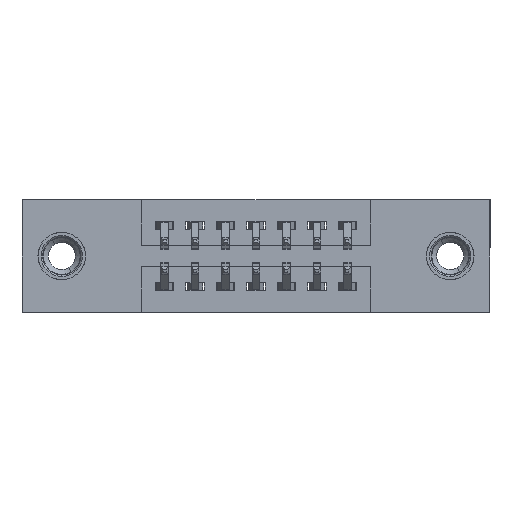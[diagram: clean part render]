
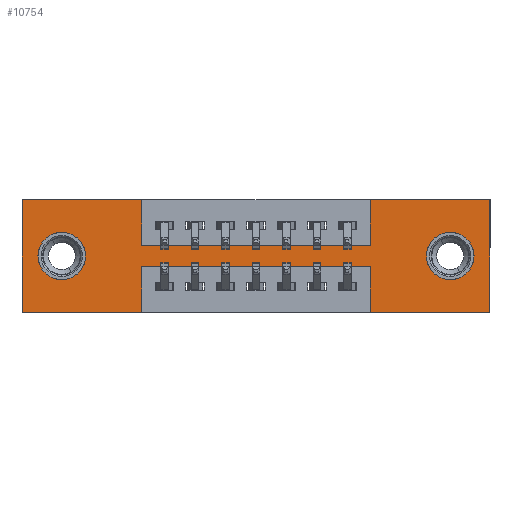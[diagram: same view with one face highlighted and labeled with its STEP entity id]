
A CAD part, front view. The second image highlights one B-rep face of the part: STEP entity #10754.
In plain terms, the highlighted planar face has unit normal (0, -1, 0).
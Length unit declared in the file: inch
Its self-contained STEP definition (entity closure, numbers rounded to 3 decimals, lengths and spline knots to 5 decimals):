
#37 = DIRECTION ( 'NONE',  ( 0., 1., 0. ) ) ;
#126 = DIRECTION ( 'NONE',  ( 0., 0., 1. ) ) ;
#140 = CARTESIAN_POINT ( 'NONE',  ( 0., 0., -0.37 ) ) ;
#160 = CARTESIAN_POINT ( 'NONE',  ( 1.1425, 0., -0.37 ) ) ;
#233 = VERTEX_POINT ( 'NONE', #1123 ) ;
#280 = DIRECTION ( 'NONE',  ( 0., 0., -1. ) ) ;
#320 = LINE ( 'NONE', #11896, #3684 ) ;
#445 = ORIENTED_EDGE ( 'NONE', *, *, #13156, .F. ) ;
#473 = ORIENTED_EDGE ( 'NONE', *, *, #13990, .F. ) ;
#594 = VECTOR ( 'NONE', #12571, 39.37008 ) ;
#724 = VERTEX_POINT ( 'NONE', #12053 ) ;
#751 = EDGE_LOOP ( 'NONE', ( #2129, #831 ) ) ;
#767 = ORIENTED_EDGE ( 'NONE', *, *, #3498, .T. ) ;
#792 = CARTESIAN_POINT ( 'NONE',  ( 0.3925, 0., -0.37 ) ) ;
#831 = ORIENTED_EDGE ( 'NONE', *, *, #5526, .T. ) ;
#1032 = ORIENTED_EDGE ( 'NONE', *, *, #11432, .F. ) ;
#1123 = CARTESIAN_POINT ( 'NONE',  ( 1.1425, 0., -0.15 ) ) ;
#1254 = CARTESIAN_POINT ( 'NONE',  ( 0., 0., 0. ) ) ;
#1284 = ORIENTED_EDGE ( 'NONE', *, *, #15122, .F. ) ;
#1580 = LINE ( 'NONE', #1654, #10946 ) ;
#1654 = CARTESIAN_POINT ( 'NONE',  ( 0.3925, 0., -0.22 ) ) ;
#1735 = LINE ( 'NONE', #140, #10733 ) ;
#1792 = VERTEX_POINT ( 'NONE', #6882 ) ;
#1902 = CARTESIAN_POINT ( 'NONE',  ( 0.3925, 0., 0. ) ) ;
#2129 = ORIENTED_EDGE ( 'NONE', *, *, #14119, .T. ) ;
#2216 = AXIS2_PLACEMENT_3D ( 'NONE', #4297, #10157, #3163 ) ;
#2231 = EDGE_CURVE ( 'NONE', #6655, #9765, #9321, .T. ) ;
#2238 = ORIENTED_EDGE ( 'NONE', *, *, #10975, .F. ) ;
#2498 = VECTOR ( 'NONE', #12984, 39.37008 ) ;
#2503 = VERTEX_POINT ( 'NONE', #13087 ) ;
#2559 = VERTEX_POINT ( 'NONE', #5867 ) ;
#2939 = LINE ( 'NONE', #14833, #11498 ) ;
#3027 = CARTESIAN_POINT ( 'NONE',  ( 0., 0., 0. ) ) ;
#3074 = EDGE_CURVE ( 'NONE', #1792, #12437, #1735, .T. ) ;
#3163 = DIRECTION ( 'NONE',  ( 0., 0., -1. ) ) ;
#3257 = LINE ( 'NONE', #14466, #6117 ) ;
#3259 = ORIENTED_EDGE ( 'NONE', *, *, #11015, .T. ) ;
#3344 = CARTESIAN_POINT ( 'NONE',  ( 0.13, 0., -0.263 ) ) ;
#3498 = EDGE_CURVE ( 'NONE', #9785, #724, #6095, .T. ) ;
#3549 = VECTOR ( 'NONE', #12951, 39.37008 ) ;
#3595 = ORIENTED_EDGE ( 'NONE', *, *, #13204, .F. ) ;
#3684 = VECTOR ( 'NONE', #5049, 39.37008 ) ;
#3766 = FACE_BOUND ( 'NONE', #751, .T. ) ;
#3791 = EDGE_CURVE ( 'NONE', #233, #10198, #3257, .T. ) ;
#4177 = CARTESIAN_POINT ( 'NONE',  ( 0.3925, 0., -0.15 ) ) ;
#4223 = DIRECTION ( 'NONE',  ( 0., 1., 0. ) ) ;
#4297 = CARTESIAN_POINT ( 'NONE',  ( 0., 0., -0.37 ) ) ;
#4320 = LINE ( 'NONE', #10291, #594 ) ;
#4828 = CARTESIAN_POINT ( 'NONE',  ( 1.1425, 0., -0.37 ) ) ;
#4930 = CARTESIAN_POINT ( 'NONE',  ( 0.13, 0., -0.185 ) ) ;
#4999 = ORIENTED_EDGE ( 'NONE', *, *, #3074, .F. ) ;
#5049 = DIRECTION ( 'NONE',  ( 0., 0., -1. ) ) ;
#5526 = EDGE_CURVE ( 'NONE', #5575, #7166, #11406, .T. ) ;
#5575 = VERTEX_POINT ( 'NONE', #7829 ) ;
#5647 = CARTESIAN_POINT ( 'NONE',  ( 0., 0., 0. ) ) ;
#5775 = CARTESIAN_POINT ( 'NONE',  ( 1.405, 0., -0.107 ) ) ;
#5867 = CARTESIAN_POINT ( 'NONE',  ( 1.535, 0., -0.37 ) ) ;
#6095 = CIRCLE ( 'NONE', #7546, 0.078 ) ;
#6117 = VECTOR ( 'NONE', #11138, 39.37008 ) ;
#6133 = DIRECTION ( 'NONE',  ( 0., 0., 1. ) ) ;
#6165 = VECTOR ( 'NONE', #9163, 39.37008 ) ;
#6533 = AXIS2_PLACEMENT_3D ( 'NONE', #14329, #7609, #280 ) ;
#6598 = LINE ( 'NONE', #792, #6165 ) ;
#6655 = VERTEX_POINT ( 'NONE', #4828 ) ;
#6708 = DIRECTION ( 'NONE',  ( 0., 0., -1. ) ) ;
#6790 = DIRECTION ( 'NONE',  ( -1., 0., 0. ) ) ;
#6882 = CARTESIAN_POINT ( 'NONE',  ( 0.3925, 0., -0.37 ) ) ;
#6951 = FACE_BOUND ( 'NONE', #11515, .T. ) ;
#7166 = VERTEX_POINT ( 'NONE', #5775 ) ;
#7375 = AXIS2_PLACEMENT_3D ( 'NONE', #11141, #4223, #12263 ) ;
#7396 = CARTESIAN_POINT ( 'NONE',  ( 0.13, 0., -0.185 ) ) ;
#7546 = AXIS2_PLACEMENT_3D ( 'NONE', #4930, #12903, #6133 ) ;
#7609 = DIRECTION ( 'NONE',  ( 0., 1., 0. ) ) ;
#7813 = DIRECTION ( 'NONE',  ( 1., 0., 0. ) ) ;
#7829 = CARTESIAN_POINT ( 'NONE',  ( 1.405, 0., -0.263 ) ) ;
#8384 = CARTESIAN_POINT ( 'NONE',  ( 1.535, 0., 0. ) ) ;
#8513 = VERTEX_POINT ( 'NONE', #4177 ) ;
#8518 = DIRECTION ( 'NONE',  ( 0., 0., 1. ) ) ;
#8630 = VECTOR ( 'NONE', #126, 39.37008 ) ;
#8665 = VECTOR ( 'NONE', #6708, 39.37008 ) ;
#8810 = VERTEX_POINT ( 'NONE', #8384 ) ;
#8982 = CARTESIAN_POINT ( 'NONE',  ( 1.1425, 0., 0. ) ) ;
#9163 = DIRECTION ( 'NONE',  ( 0., 0., -1. ) ) ;
#9321 = LINE ( 'NONE', #160, #8630 ) ;
#9758 = LINE ( 'NONE', #1254, #3549 ) ;
#9765 = VERTEX_POINT ( 'NONE', #13679 ) ;
#9785 = VERTEX_POINT ( 'NONE', #3344 ) ;
#9891 = ORIENTED_EDGE ( 'NONE', *, *, #13495, .F. ) ;
#9950 = FACE_OUTER_BOUND ( 'NONE', #11620, .T. ) ;
#10157 = DIRECTION ( 'NONE',  ( 0., -1., 0. ) ) ;
#10166 = EDGE_CURVE ( 'NONE', #10230, #10204, #14355, .T. ) ;
#10198 = VERTEX_POINT ( 'NONE', #8982 ) ;
#10204 = VERTEX_POINT ( 'NONE', #1902 ) ;
#10230 = VERTEX_POINT ( 'NONE', #5647 ) ;
#10291 = CARTESIAN_POINT ( 'NONE',  ( 0., 0., -0.37 ) ) ;
#10733 = VECTOR ( 'NONE', #6790, 39.37008 ) ;
#10754 = ADVANCED_FACE ( 'NONE', ( #3766, #6951, #9950 ), #14640, .T. ) ;
#10946 = VECTOR ( 'NONE', #13266, 39.37008 ) ;
#10975 = EDGE_CURVE ( 'NONE', #10198, #8810, #9758, .T. ) ;
#11015 = EDGE_CURVE ( 'NONE', #724, #9785, #12742, .T. ) ;
#11109 = CIRCLE ( 'NONE', #6533, 0.078 ) ;
#11138 = DIRECTION ( 'NONE',  ( 0., 0., 1. ) ) ;
#11141 = CARTESIAN_POINT ( 'NONE',  ( 1.405, 0., -0.185 ) ) ;
#11406 = CIRCLE ( 'NONE', #7375, 0.078 ) ;
#11432 = EDGE_CURVE ( 'NONE', #2559, #6655, #4320, .T. ) ;
#11498 = VECTOR ( 'NONE', #12566, 39.37008 ) ;
#11515 = EDGE_LOOP ( 'NONE', ( #3259, #767 ) ) ;
#11620 = EDGE_LOOP ( 'NONE', ( #3595, #9891, #11717, #1032, #473, #2238, #12476, #12797, #445, #13026, #1284, #4999 ) ) ;
#11717 = ORIENTED_EDGE ( 'NONE', *, *, #2231, .F. ) ;
#11896 = CARTESIAN_POINT ( 'NONE',  ( 1.535, 0., 0. ) ) ;
#12053 = CARTESIAN_POINT ( 'NONE',  ( 0.13, 0., -0.107 ) ) ;
#12263 = DIRECTION ( 'NONE',  ( 0., 0., -1. ) ) ;
#12437 = VERTEX_POINT ( 'NONE', #14450 ) ;
#12471 = CARTESIAN_POINT ( 'NONE',  ( 0.3925, 0., 0. ) ) ;
#12476 = ORIENTED_EDGE ( 'NONE', *, *, #3791, .F. ) ;
#12566 = DIRECTION ( 'NONE',  ( 1., 0., 0. ) ) ;
#12571 = DIRECTION ( 'NONE',  ( -1., 0., 0. ) ) ;
#12742 = CIRCLE ( 'NONE', #13116, 0.078 ) ;
#12797 = ORIENTED_EDGE ( 'NONE', *, *, #13251, .F. ) ;
#12903 = DIRECTION ( 'NONE',  ( 0., 1., 0. ) ) ;
#12951 = DIRECTION ( 'NONE',  ( 1., 0., 0. ) ) ;
#12984 = DIRECTION ( 'NONE',  ( 0., 0., 1. ) ) ;
#13026 = ORIENTED_EDGE ( 'NONE', *, *, #10166, .F. ) ;
#13087 = CARTESIAN_POINT ( 'NONE',  ( 0.3925, 0., -0.22 ) ) ;
#13116 = AXIS2_PLACEMENT_3D ( 'NONE', #7396, #37, #8518 ) ;
#13156 = EDGE_CURVE ( 'NONE', #10204, #8513, #14661, .T. ) ;
#13204 = EDGE_CURVE ( 'NONE', #2503, #1792, #6598, .T. ) ;
#13251 = EDGE_CURVE ( 'NONE', #8513, #233, #2939, .T. ) ;
#13266 = DIRECTION ( 'NONE',  ( -1., 0., 0. ) ) ;
#13495 = EDGE_CURVE ( 'NONE', #9765, #2503, #1580, .T. ) ;
#13679 = CARTESIAN_POINT ( 'NONE',  ( 1.1425, 0., -0.22 ) ) ;
#13713 = LINE ( 'NONE', #14066, #2498 ) ;
#13990 = EDGE_CURVE ( 'NONE', #8810, #2559, #320, .T. ) ;
#14024 = VECTOR ( 'NONE', #7813, 39.37008 ) ;
#14066 = CARTESIAN_POINT ( 'NONE',  ( 0., 0., 0. ) ) ;
#14119 = EDGE_CURVE ( 'NONE', #7166, #5575, #11109, .T. ) ;
#14329 = CARTESIAN_POINT ( 'NONE',  ( 1.405, 0., -0.185 ) ) ;
#14355 = LINE ( 'NONE', #3027, #14024 ) ;
#14450 = CARTESIAN_POINT ( 'NONE',  ( 0., 0., -0.37 ) ) ;
#14466 = CARTESIAN_POINT ( 'NONE',  ( 1.1425, 0., 0. ) ) ;
#14640 = PLANE ( 'NONE',  #2216 ) ;
#14661 = LINE ( 'NONE', #12471, #8665 ) ;
#14833 = CARTESIAN_POINT ( 'NONE',  ( 0.3925, 0., -0.15 ) ) ;
#15122 = EDGE_CURVE ( 'NONE', #12437, #10230, #13713, .T. ) ;
